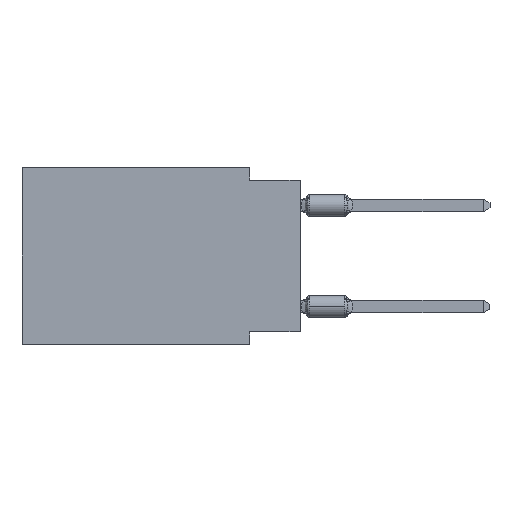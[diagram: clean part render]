
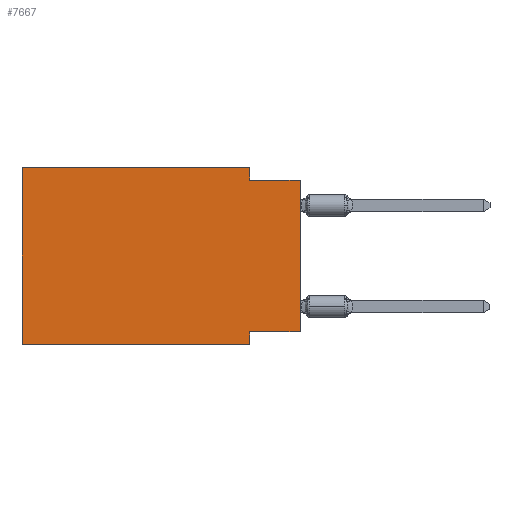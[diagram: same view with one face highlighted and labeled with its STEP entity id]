
A CAD part, left-side view. The second image highlights one B-rep face of the part: STEP entity #7667.
In plain terms, the highlighted planar face has unit normal (-1, 0, 0).
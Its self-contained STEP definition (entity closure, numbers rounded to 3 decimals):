
#315 = ORIENTED_EDGE ( 'NONE', *, *, #9468, .F. ) ;
#399 = CARTESIAN_POINT ( 'NONE',  ( 0., 0., -8.255 ) ) ;
#757 = VECTOR ( 'NONE', #3913, 1000. ) ;
#876 = AXIS2_PLACEMENT_3D ( 'NONE', #7959, #12105, #8025 ) ;
#1041 = DIRECTION ( 'NONE',  ( 0., 0., 1. ) ) ;
#1204 = VERTEX_POINT ( 'NONE', #399 ) ;
#1465 = VERTEX_POINT ( 'NONE', #4949 ) ;
#1967 = EDGE_CURVE ( 'NONE', #6398, #1465, #1994, .T. ) ;
#1994 = LINE ( 'NONE', #7179, #757 ) ;
#2186 = ORIENTED_EDGE ( 'NONE', *, *, #2804, .T. ) ;
#2271 = ORIENTED_EDGE ( 'NONE', *, *, #12750, .F. ) ;
#2507 = LINE ( 'NONE', #10962, #8968 ) ;
#2605 = LINE ( 'NONE', #5748, #12779 ) ;
#2779 = LINE ( 'NONE', #7148, #4460 ) ;
#2804 = EDGE_CURVE ( 'NONE', #11265, #12727, #2779, .T. ) ;
#3232 = ORIENTED_EDGE ( 'NONE', *, *, #10034, .F. ) ;
#3365 = ORIENTED_EDGE ( 'NONE', *, *, #8154, .F. ) ;
#3430 = CARTESIAN_POINT ( 'NONE',  ( 0., 2.54, 0. ) ) ;
#3439 = LINE ( 'NONE', #11763, #7085 ) ;
#3913 = DIRECTION ( 'NONE',  ( 0., -1., 0. ) ) ;
#3945 = EDGE_CURVE ( 'NONE', #7942, #4711, #2507, .T. ) ;
#3963 = DIRECTION ( 'NONE',  ( 0., 0., -1. ) ) ;
#4460 = VECTOR ( 'NONE', #6129, 1000. ) ;
#4711 = VERTEX_POINT ( 'NONE', #3430 ) ;
#4949 = CARTESIAN_POINT ( 'NONE',  ( 0., 0., -0.635 ) ) ;
#5339 = CARTESIAN_POINT ( 'NONE',  ( 0., 0., 0. ) ) ;
#5685 = CARTESIAN_POINT ( 'NONE',  ( 0., 13.97, 0. ) ) ;
#5748 = CARTESIAN_POINT ( 'NONE',  ( 0., 0., -8.255 ) ) ;
#5864 = DIRECTION ( 'NONE',  ( 0., -1., 0. ) ) ;
#5908 = PLANE ( 'NONE',  #876 ) ;
#6129 = DIRECTION ( 'NONE',  ( 0., -1., 0. ) ) ;
#6221 = CARTESIAN_POINT ( 'NONE',  ( 0., 13.97, -8.89 ) ) ;
#6398 = VERTEX_POINT ( 'NONE', #6857 ) ;
#6857 = CARTESIAN_POINT ( 'NONE',  ( 0., 2.54, -0.635 ) ) ;
#7085 = VECTOR ( 'NONE', #7745, 1000. ) ;
#7096 = CARTESIAN_POINT ( 'NONE',  ( 0., 2.54, -8.89 ) ) ;
#7148 = CARTESIAN_POINT ( 'NONE',  ( 0., 13.97, -8.89 ) ) ;
#7179 = CARTESIAN_POINT ( 'NONE',  ( 0., 0., -0.635 ) ) ;
#7305 = CARTESIAN_POINT ( 'NONE',  ( 0., 13.97, 0. ) ) ;
#7333 = VERTEX_POINT ( 'NONE', #7480 ) ;
#7375 = DIRECTION ( 'NONE',  ( 0., 0., 1. ) ) ;
#7480 = CARTESIAN_POINT ( 'NONE',  ( 0., 2.54, -8.255 ) ) ;
#7667 = ADVANCED_FACE ( 'NONE', ( #13264 ), #5908, .F. ) ;
#7745 = DIRECTION ( 'NONE',  ( 0., 0., -1. ) ) ;
#7757 = ORIENTED_EDGE ( 'NONE', *, *, #3945, .F. ) ;
#7942 = VERTEX_POINT ( 'NONE', #5685 ) ;
#7959 = CARTESIAN_POINT ( 'NONE',  ( 0., 13.97, 0. ) ) ;
#8002 = ORIENTED_EDGE ( 'NONE', *, *, #8174, .T. ) ;
#8025 = DIRECTION ( 'NONE',  ( 0., 0., -1. ) ) ;
#8154 = EDGE_CURVE ( 'NONE', #1204, #7333, #2605, .T. ) ;
#8174 = EDGE_CURVE ( 'NONE', #1204, #1465, #11532, .T. ) ;
#8671 = VECTOR ( 'NONE', #7375, 1000. ) ;
#8826 = ORIENTED_EDGE ( 'NONE', *, *, #1967, .F. ) ;
#8968 = VECTOR ( 'NONE', #5864, 1000. ) ;
#9468 = EDGE_CURVE ( 'NONE', #7333, #12727, #3439, .T. ) ;
#9639 = EDGE_LOOP ( 'NONE', ( #8002, #8826, #2271, #7757, #3232, #2186, #315, #3365 ) ) ;
#9901 = DIRECTION ( 'NONE',  ( 0., 1., 0. ) ) ;
#9964 = VECTOR ( 'NONE', #3963, 1000. ) ;
#10034 = EDGE_CURVE ( 'NONE', #11265, #7942, #12547, .T. ) ;
#10962 = CARTESIAN_POINT ( 'NONE',  ( 0., 13.97, 0. ) ) ;
#11265 = VERTEX_POINT ( 'NONE', #6221 ) ;
#11319 = LINE ( 'NONE', #12073, #9964 ) ;
#11532 = LINE ( 'NONE', #5339, #8671 ) ;
#11763 = CARTESIAN_POINT ( 'NONE',  ( 0., 2.54, -8.89 ) ) ;
#12073 = CARTESIAN_POINT ( 'NONE',  ( 0., 2.54, 0. ) ) ;
#12105 = DIRECTION ( 'NONE',  ( 1., 0., 0. ) ) ;
#12547 = LINE ( 'NONE', #7305, #12958 ) ;
#12727 = VERTEX_POINT ( 'NONE', #7096 ) ;
#12750 = EDGE_CURVE ( 'NONE', #4711, #6398, #11319, .T. ) ;
#12779 = VECTOR ( 'NONE', #9901, 1000. ) ;
#12958 = VECTOR ( 'NONE', #1041, 1000. ) ;
#13264 = FACE_OUTER_BOUND ( 'NONE', #9639, .T. ) ;
